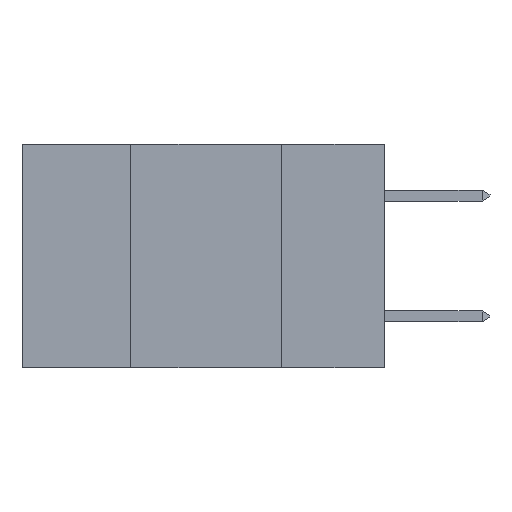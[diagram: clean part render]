
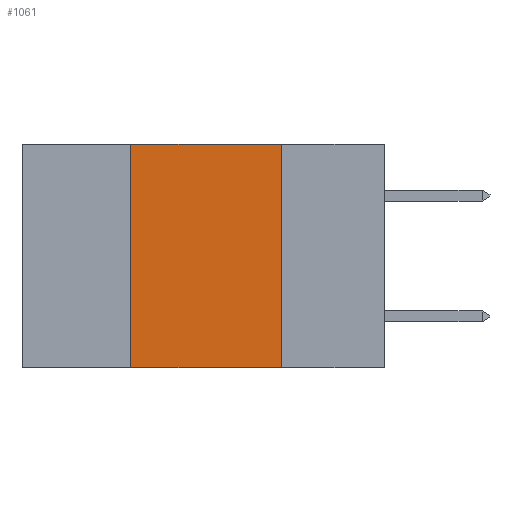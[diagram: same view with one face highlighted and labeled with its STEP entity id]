
A CAD part, left-side view. The second image highlights one B-rep face of the part: STEP entity #1061.
In plain terms, the highlighted planar face has unit normal (-1, 0, 0).
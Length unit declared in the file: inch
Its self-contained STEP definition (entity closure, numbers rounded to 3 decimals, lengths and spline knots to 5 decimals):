
#546 = LINE ( 'NONE', #7516, #6185 ) ;
#776 = VERTEX_POINT ( 'NONE', #9644 ) ;
#1061 = ADVANCED_FACE ( 'NONE', ( #1855 ), #6194, .F. ) ;
#1455 = VERTEX_POINT ( 'NONE', #5559 ) ;
#1825 = VECTOR ( 'NONE', #3073, 39.37008 ) ;
#1854 = EDGE_LOOP ( 'NONE', ( #12272, #3844, #7134, #5655 ) ) ;
#1855 = FACE_OUTER_BOUND ( 'NONE', #1854, .T. ) ;
#1988 = EDGE_CURVE ( 'NONE', #776, #4700, #10162, .T. ) ;
#3073 = DIRECTION ( 'NONE',  ( 0., 0., -1. ) ) ;
#3844 = ORIENTED_EDGE ( 'NONE', *, *, #11254, .F. ) ;
#4194 = VERTEX_POINT ( 'NONE', #9922 ) ;
#4460 = DIRECTION ( 'NONE',  ( 1., 0., 0. ) ) ;
#4513 = CARTESIAN_POINT ( 'NONE',  ( 0., 0.17, -0.37 ) ) ;
#4700 = VERTEX_POINT ( 'NONE', #4513 ) ;
#4850 = CARTESIAN_POINT ( 'NONE',  ( 0., 0.6, 0. ) ) ;
#5223 = LINE ( 'NONE', #12188, #13178 ) ;
#5559 = CARTESIAN_POINT ( 'NONE',  ( 0., 0.42, -0.37 ) ) ;
#5655 = ORIENTED_EDGE ( 'NONE', *, *, #7520, .T. ) ;
#5838 = LINE ( 'NONE', #7126, #11003 ) ;
#5878 = EDGE_CURVE ( 'NONE', #1455, #4194, #546, .T. ) ;
#6185 = VECTOR ( 'NONE', #11658, 39.37008 ) ;
#6194 = PLANE ( 'NONE',  #12767 ) ;
#7126 = CARTESIAN_POINT ( 'NONE',  ( 0., 0.6, -0.37 ) ) ;
#7134 = ORIENTED_EDGE ( 'NONE', *, *, #5878, .F. ) ;
#7516 = CARTESIAN_POINT ( 'NONE',  ( 0., 0.42, 0. ) ) ;
#7520 = EDGE_CURVE ( 'NONE', #1455, #4700, #5838, .T. ) ;
#9295 = CARTESIAN_POINT ( 'NONE',  ( 0., 0.17, 0. ) ) ;
#9644 = CARTESIAN_POINT ( 'NONE',  ( 0., 0.17, 0. ) ) ;
#9922 = CARTESIAN_POINT ( 'NONE',  ( 0., 0.42, 0. ) ) ;
#10162 = LINE ( 'NONE', #9295, #1825 ) ;
#11003 = VECTOR ( 'NONE', #13311, 39.37008 ) ;
#11254 = EDGE_CURVE ( 'NONE', #4194, #776, #5223, .T. ) ;
#11658 = DIRECTION ( 'NONE',  ( 0., 0., 1. ) ) ;
#12188 = CARTESIAN_POINT ( 'NONE',  ( 0., 0.6, 0. ) ) ;
#12272 = ORIENTED_EDGE ( 'NONE', *, *, #1988, .F. ) ;
#12499 = DIRECTION ( 'NONE',  ( 0., 0., -1. ) ) ;
#12767 = AXIS2_PLACEMENT_3D ( 'NONE', #4850, #4460, #12499 ) ;
#13178 = VECTOR ( 'NONE', #13243, 39.37008 ) ;
#13243 = DIRECTION ( 'NONE',  ( 0., -1., 0. ) ) ;
#13311 = DIRECTION ( 'NONE',  ( 0., -1., 0. ) ) ;
